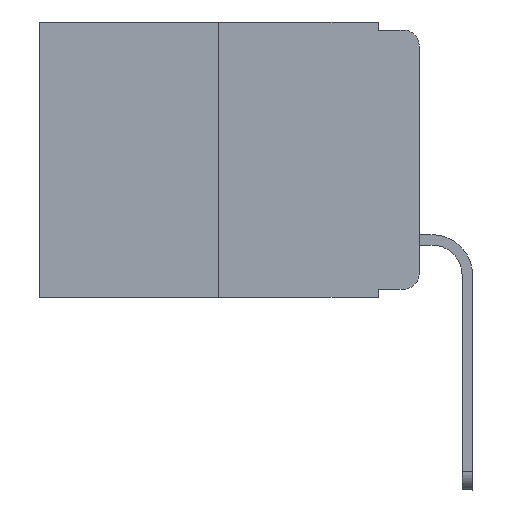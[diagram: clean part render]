
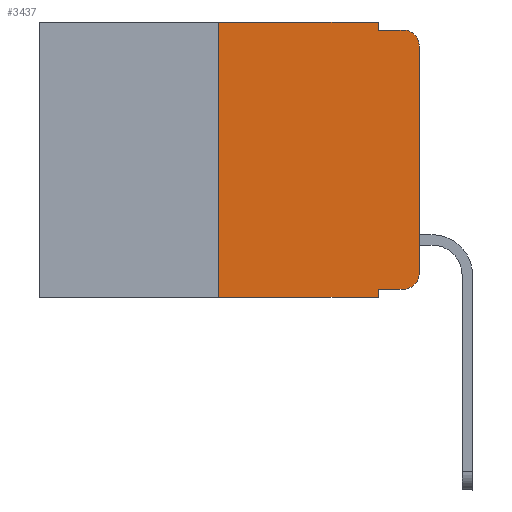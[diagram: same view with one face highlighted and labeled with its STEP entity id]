
A CAD part, left-side view. The second image highlights one B-rep face of the part: STEP entity #3437.
In plain terms, the highlighted planar face has unit normal (-1, 0, 0).
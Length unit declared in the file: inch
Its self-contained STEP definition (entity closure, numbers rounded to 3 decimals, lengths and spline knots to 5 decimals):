
#10 = CARTESIAN_POINT ( 'NONE',  ( 0., 0.051, -0.333 ) ) ;
#48 = DIRECTION ( 'NONE',  ( 0., -1., 0. ) ) ;
#657 = CARTESIAN_POINT ( 'NONE',  ( 0., 0.473, 0. ) ) ;
#750 = EDGE_CURVE ( 'NONE', #3269, #9633, #7648, .T. ) ;
#766 = LINE ( 'NONE', #4300, #6650 ) ;
#1112 = LINE ( 'NONE', #10175, #8519 ) ;
#1226 = CARTESIAN_POINT ( 'NONE',  ( 0., 0.051, 0. ) ) ;
#1440 = LINE ( 'NONE', #8127, #9484 ) ;
#1488 = EDGE_CURVE ( 'NONE', #3397, #10731, #8754, .T. ) ;
#1834 = VERTEX_POINT ( 'NONE', #10844 ) ;
#1851 = ORIENTED_EDGE ( 'NONE', *, *, #6444, .F. ) ;
#1972 = CARTESIAN_POINT ( 'NONE',  ( 0., 0.051, 0. ) ) ;
#1984 = VECTOR ( 'NONE', #2947, 39.37008 ) ;
#2182 = DIRECTION ( 'NONE',  ( -1., 0., 0. ) ) ;
#2240 = CIRCLE ( 'NONE', #9436, 0.02 ) ;
#2364 = FACE_OUTER_BOUND ( 'NONE', #10671, .T. ) ;
#2401 = ORIENTED_EDGE ( 'NONE', *, *, #8113, .T. ) ;
#2552 = LINE ( 'NONE', #3507, #3160 ) ;
#2555 = EDGE_CURVE ( 'NONE', #1834, #4890, #3138, .T. ) ;
#2630 = CARTESIAN_POINT ( 'NONE',  ( 0., 0.02, -0.333 ) ) ;
#2780 = AXIS2_PLACEMENT_3D ( 'NONE', #657, #10650, #4928 ) ;
#2887 = AXIS2_PLACEMENT_3D ( 'NONE', #4769, #4716, #8138 ) ;
#2947 = DIRECTION ( 'NONE',  ( 0., 0., -1. ) ) ;
#3138 = LINE ( 'NONE', #10, #5027 ) ;
#3146 = VERTEX_POINT ( 'NONE', #9353 ) ;
#3160 = VECTOR ( 'NONE', #5908, 39.37008 ) ;
#3269 = VERTEX_POINT ( 'NONE', #6209 ) ;
#3397 = VERTEX_POINT ( 'NONE', #1972 ) ;
#3437 = ADVANCED_FACE ( 'NONE', ( #2364 ), #4704, .F. ) ;
#3507 = CARTESIAN_POINT ( 'NONE',  ( 0., 0.473, 0. ) ) ;
#3768 = VECTOR ( 'NONE', #3779, 39.37008 ) ;
#3779 = DIRECTION ( 'NONE',  ( 0., 0., -1. ) ) ;
#3840 = VERTEX_POINT ( 'NONE', #7412 ) ;
#3854 = ORIENTED_EDGE ( 'NONE', *, *, #3997, .F. ) ;
#3997 = EDGE_CURVE ( 'NONE', #9756, #3146, #766, .T. ) ;
#4300 = CARTESIAN_POINT ( 'NONE',  ( 0., 0.25, 0. ) ) ;
#4704 = PLANE ( 'NONE',  #2780 ) ;
#4716 = DIRECTION ( 'NONE',  ( -1., 0., 0. ) ) ;
#4769 = CARTESIAN_POINT ( 'NONE',  ( 0., 0.02, -0.03 ) ) ;
#4890 = VERTEX_POINT ( 'NONE', #2630 ) ;
#4928 = DIRECTION ( 'NONE',  ( 0., 0., -1. ) ) ;
#4941 = CARTESIAN_POINT ( 'NONE',  ( 0., 0.051, -0.01 ) ) ;
#4952 = ORIENTED_EDGE ( 'NONE', *, *, #1488, .F. ) ;
#4978 = DIRECTION ( 'NONE',  ( 0., 0., 1. ) ) ;
#4981 = VECTOR ( 'NONE', #8382, 39.37008 ) ;
#5027 = VECTOR ( 'NONE', #10739, 39.37008 ) ;
#5701 = CARTESIAN_POINT ( 'NONE',  ( 0., 0.02, -0.313 ) ) ;
#5908 = DIRECTION ( 'NONE',  ( 0., -1., 0. ) ) ;
#6209 = CARTESIAN_POINT ( 'NONE',  ( 0., 0., -0.03 ) ) ;
#6444 = EDGE_CURVE ( 'NONE', #1834, #3840, #9010, .T. ) ;
#6468 = ORIENTED_EDGE ( 'NONE', *, *, #2555, .T. ) ;
#6548 = ORIENTED_EDGE ( 'NONE', *, *, #7535, .F. ) ;
#6650 = VECTOR ( 'NONE', #4978, 39.37008 ) ;
#7350 = DIRECTION ( 'NONE',  ( 0., 0., -1. ) ) ;
#7412 = CARTESIAN_POINT ( 'NONE',  ( 0., 0.051, -0.343 ) ) ;
#7535 = EDGE_CURVE ( 'NONE', #3146, #3397, #2552, .T. ) ;
#7648 = CIRCLE ( 'NONE', #2887, 0.02 ) ;
#8113 = EDGE_CURVE ( 'NONE', #4890, #9758, #2240, .T. ) ;
#8127 = CARTESIAN_POINT ( 'NONE',  ( 0., 0.473, -0.343 ) ) ;
#8138 = DIRECTION ( 'NONE',  ( 0., 0., -1. ) ) ;
#8382 = DIRECTION ( 'NONE',  ( 0., 0., 1. ) ) ;
#8484 = CARTESIAN_POINT ( 'NONE',  ( 0., 0., 0. ) ) ;
#8519 = VECTOR ( 'NONE', #48, 39.37008 ) ;
#8754 = LINE ( 'NONE', #1226, #3768 ) ;
#8834 = CARTESIAN_POINT ( 'NONE',  ( 0., 0.02, -0.01 ) ) ;
#9010 = LINE ( 'NONE', #10481, #1984 ) ;
#9261 = LINE ( 'NONE', #8484, #4981 ) ;
#9321 = EDGE_CURVE ( 'NONE', #10731, #9633, #1112, .T. ) ;
#9353 = CARTESIAN_POINT ( 'NONE',  ( 0., 0.25, 0. ) ) ;
#9436 = AXIS2_PLACEMENT_3D ( 'NONE', #5701, #2182, #7350 ) ;
#9484 = VECTOR ( 'NONE', #10652, 39.37008 ) ;
#9573 = EDGE_CURVE ( 'NONE', #9756, #3840, #1440, .T. ) ;
#9633 = VERTEX_POINT ( 'NONE', #8834 ) ;
#9756 = VERTEX_POINT ( 'NONE', #10576 ) ;
#9758 = VERTEX_POINT ( 'NONE', #10693 ) ;
#9928 = ORIENTED_EDGE ( 'NONE', *, *, #750, .T. ) ;
#10012 = ORIENTED_EDGE ( 'NONE', *, *, #9573, .T. ) ;
#10057 = ORIENTED_EDGE ( 'NONE', *, *, #9321, .F. ) ;
#10171 = ORIENTED_EDGE ( 'NONE', *, *, #10343, .T. ) ;
#10175 = CARTESIAN_POINT ( 'NONE',  ( 0., 0.051, -0.01 ) ) ;
#10343 = EDGE_CURVE ( 'NONE', #9758, #3269, #9261, .T. ) ;
#10481 = CARTESIAN_POINT ( 'NONE',  ( 0., 0.051, 0. ) ) ;
#10576 = CARTESIAN_POINT ( 'NONE',  ( 0., 0.25, -0.343 ) ) ;
#10650 = DIRECTION ( 'NONE',  ( 1., 0., 0. ) ) ;
#10652 = DIRECTION ( 'NONE',  ( 0., -1., 0. ) ) ;
#10671 = EDGE_LOOP ( 'NONE', ( #10171, #9928, #10057, #4952, #6548, #3854, #10012, #1851, #6468, #2401 ) ) ;
#10693 = CARTESIAN_POINT ( 'NONE',  ( 0., 0., -0.313 ) ) ;
#10731 = VERTEX_POINT ( 'NONE', #4941 ) ;
#10739 = DIRECTION ( 'NONE',  ( 0., -1., 0. ) ) ;
#10844 = CARTESIAN_POINT ( 'NONE',  ( 0., 0.051, -0.333 ) ) ;
